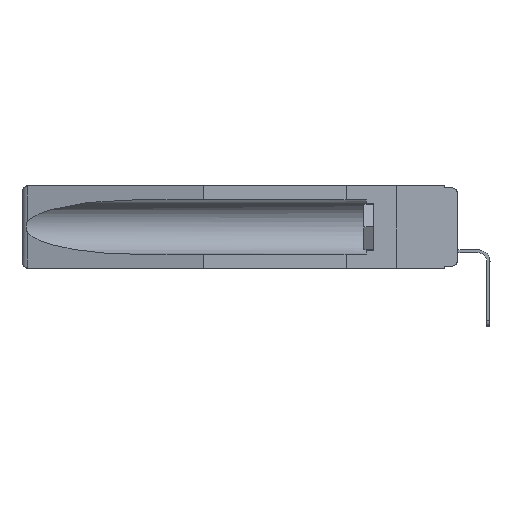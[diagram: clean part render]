
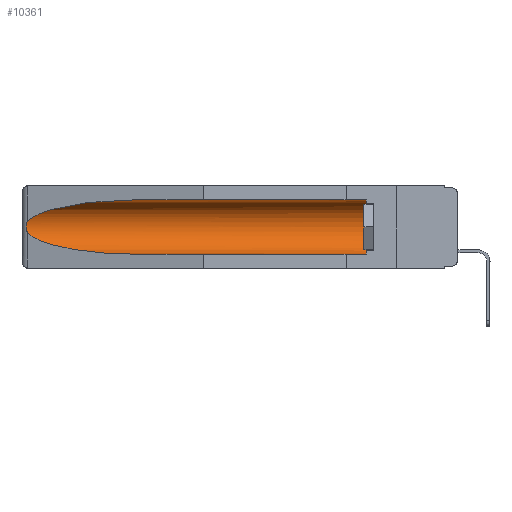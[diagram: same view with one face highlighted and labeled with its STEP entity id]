
A CAD part, left-side view. The second image highlights one B-rep face of the part: STEP entity #10361.
In plain terms, the highlighted cylindrical face has radius 2.857 mm (diameter 5.715 mm), a partial arc.
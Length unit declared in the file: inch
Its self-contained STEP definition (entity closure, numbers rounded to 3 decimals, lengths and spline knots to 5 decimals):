
#53 = DIRECTION ( 'NONE',  ( 0., 1., 0. ) ) ;
#136 = LINE ( 'NONE', #20143, #1429 ) ;
#909 = CARTESIAN_POINT ( 'NONE',  ( 0.26537, 1.52718, -0.14972 ) ) ;
#952 = CARTESIAN_POINT ( 'NONE',  ( 0.21114, 1.30732, -0.284 ) ) ;
#1034 = CARTESIAN_POINT ( 'NONE',  ( 0.26537, 1.52718, -0.19328 ) ) ;
#1062 = FACE_OUTER_BOUND ( 'NONE', #20499, .T. ) ;
#1429 = VECTOR ( 'NONE', #53, 39.37008 ) ;
#2511 = CARTESIAN_POINT ( 'NONE',  ( 0.155, 1.07973, -0.059 ) ) ;
#2600 = CARTESIAN_POINT ( 'NONE',  ( 0.2675, 1.53308, -0.16763 ) ) ;
#3013 = CARTESIAN_POINT ( 'NONE',  ( 0.26655, 1.53094, -0.18657 ) ) ;
#3169 = VERTEX_POINT ( 'NONE', #5959 ) ;
#3770 = LINE ( 'NONE', #24058, #6021 ) ;
#4301 = CARTESIAN_POINT ( 'NONE',  ( 0.21114, 1.30732, -0.059 ) ) ;
#4975 = CARTESIAN_POINT ( 'NONE',  ( 0.26597, 1.52961, -0.15275 ) ) ;
#5959 = CARTESIAN_POINT ( 'NONE',  ( 0.26537, 1.52718, -0.19328 ) ) ;
#6021 = VECTOR ( 'NONE', #12058, 39.37008 ) ;
#6102 = EDGE_CURVE ( 'NONE', #3169, #18479, #24228, .T. ) ;
#7981 = DIRECTION ( 'NONE',  ( 0., 0., 1. ) ) ;
#8430 = CARTESIAN_POINT ( 'NONE',  ( 0.26537, 1.52718, -0.14972 ) ) ;
#8599 = CARTESIAN_POINT ( 'NONE',  ( 0.2673, 1.5327, -0.16383 ) ) ;
#8892 = DIRECTION ( 'NONE',  ( 0., -1., 0. ) ) ;
#9334 = CIRCLE ( 'NONE', #17884, 0.1125 ) ;
#9586 = EDGE_CURVE ( 'NONE', #20223, #13079, #9334, .T. ) ;
#10361 = ADVANCED_FACE ( 'NONE', ( #1062 ), #22189, .F. ) ;
#11242 = CARTESIAN_POINT ( 'NONE',  ( 0.26537, 1.52718, -0.19328 ) ) ;
#11950 = DIRECTION ( 'NONE',  ( 0., 1., 0. ) ) ;
#12058 = DIRECTION ( 'NONE',  ( 0., 1., 0. ) ) ;
#13079 = VERTEX_POINT ( 'NONE', #24149 ) ;
#14222 =( BOUNDED_CURVE ( )  B_SPLINE_CURVE ( 3, ( #2511, #4301, #20469, #8430 ),
 .UNSPECIFIED., .F., .F. ) 
 B_SPLINE_CURVE_WITH_KNOTS ( ( 4, 4 ),
 ( 4.71239, 6.08839 ),
 .UNSPECIFIED. ) 
 CURVE ( )  GEOMETRIC_REPRESENTATION_ITEM ( )  RATIONAL_B_SPLINE_CURVE ( ( 1., 0.848, 0.848, 1. ) ) 
 REPRESENTATION_ITEM ( '' )  );
#14223 = ORIENTED_EDGE ( 'NONE', *, *, #25706, .T. ) ;
#14297 = ORIENTED_EDGE ( 'NONE', *, *, #15882, .F. ) ;
#14958 = DIRECTION ( 'NONE',  ( 0., 0., 1. ) ) ;
#15047 = CARTESIAN_POINT ( 'NONE',  ( 0.26537, 1.52718, -0.14972 ) ) ;
#15130 = CARTESIAN_POINT ( 'NONE',  ( 0.25451, 1.48313, -0.24835 ) ) ;
#15261 = CARTESIAN_POINT ( 'NONE',  ( 0.26597, 1.5296, -0.19026 ) ) ;
#15882 = EDGE_CURVE ( 'NONE', #20223, #18479, #3770, .T. ) ;
#16822 = CARTESIAN_POINT ( 'NONE',  ( 0.155, 0.126, -0.1715 ) ) ;
#17267 = ORIENTED_EDGE ( 'NONE', *, *, #6102, .T. ) ;
#17884 = AXIS2_PLACEMENT_3D ( 'NONE', #16822, #8892, #14958 ) ;
#18479 = VERTEX_POINT ( 'NONE', #22989 ) ;
#18941 = CARTESIAN_POINT ( 'NONE',  ( 0.155, 1.07973, -0.059 ) ) ;
#19016 = CARTESIAN_POINT ( 'NONE',  ( 0.155, 1.07973, -0.284 ) ) ;
#19058 = CARTESIAN_POINT ( 'NONE',  ( 0.26654, 1.53092, -0.15636 ) ) ;
#19684 = CARTESIAN_POINT ( 'NONE',  ( 0.155, -0.30754, -0.1715 ) ) ;
#19923 = EDGE_CURVE ( 'NONE', #13079, #21926, #136, .T. ) ;
#20140 = ORIENTED_EDGE ( 'NONE', *, *, #25928, .T. ) ;
#20143 = CARTESIAN_POINT ( 'NONE',  ( 0.155, -0.30754, -0.059 ) ) ;
#20173 = ORIENTED_EDGE ( 'NONE', *, *, #19923, .T. ) ;
#20223 = VERTEX_POINT ( 'NONE', #20911 ) ;
#20469 = CARTESIAN_POINT ( 'NONE',  ( 0.25451, 1.48313, -0.09465 ) ) ;
#20499 = EDGE_LOOP ( 'NONE', ( #14223, #20140, #17267, #14297, #22737, #20173 ) ) ;
#20911 = CARTESIAN_POINT ( 'NONE',  ( 0.155, 0.126, -0.284 ) ) ;
#21060 = AXIS2_PLACEMENT_3D ( 'NONE', #19684, #11950, #7981 ) ;
#21401 = CARTESIAN_POINT ( 'NONE',  ( 0.2673, 1.53269, -0.17917 ) ) ;
#21926 = VERTEX_POINT ( 'NONE', #18941 ) ;
#21939 = VERTEX_POINT ( 'NONE', #15047 ) ;
#21965 = B_SPLINE_CURVE_WITH_KNOTS ( 'NONE', 3,
 ( #909, #4975, #19058, #8599, #2600, #22739, #21401, #3013, #15261, #11242 ),
 .UNSPECIFIED., .F., .F.,
 ( 4, 2, 2, 2, 4 ),
 ( 0., 0.00029, 0.00058, 0.00087, 0.00117 ),
 .UNSPECIFIED. ) ;
#22189 = CYLINDRICAL_SURFACE ( 'NONE', #21060, 0.1125 ) ;
#22737 = ORIENTED_EDGE ( 'NONE', *, *, #9586, .T. ) ;
#22739 = CARTESIAN_POINT ( 'NONE',  ( 0.2675, 1.53308, -0.17534 ) ) ;
#22989 = CARTESIAN_POINT ( 'NONE',  ( 0.155, 1.07973, -0.284 ) ) ;
#24058 = CARTESIAN_POINT ( 'NONE',  ( 0.155, -0.30754, -0.284 ) ) ;
#24149 = CARTESIAN_POINT ( 'NONE',  ( 0.155, 0.126, -0.059 ) ) ;
#24228 =( BOUNDED_CURVE ( )  B_SPLINE_CURVE ( 3, ( #1034, #15130, #952, #19016 ),
 .UNSPECIFIED., .F., .F. ) 
 B_SPLINE_CURVE_WITH_KNOTS ( ( 4, 4 ),
 ( 0.1948, 1.5708 ),
 .UNSPECIFIED. ) 
 CURVE ( )  GEOMETRIC_REPRESENTATION_ITEM ( )  RATIONAL_B_SPLINE_CURVE ( ( 1., 0.848, 0.848, 1. ) ) 
 REPRESENTATION_ITEM ( '' )  );
#25706 = EDGE_CURVE ( 'NONE', #21926, #21939, #14222, .T. ) ;
#25928 = EDGE_CURVE ( 'NONE', #21939, #3169, #21965, .T. ) ;
